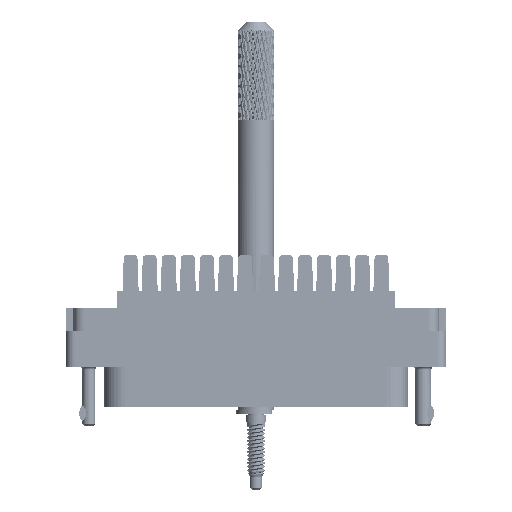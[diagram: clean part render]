
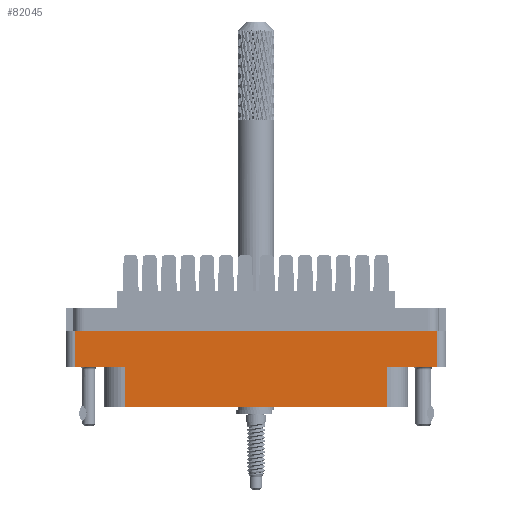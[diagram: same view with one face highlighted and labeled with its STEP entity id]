
A CAD part, front view. The second image highlights one B-rep face of the part: STEP entity #82045.
In plain terms, the highlighted planar face has unit normal (0, -1, 0).
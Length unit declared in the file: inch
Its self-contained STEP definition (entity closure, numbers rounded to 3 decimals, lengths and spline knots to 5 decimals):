
#1005 = VECTOR ( 'NONE', #51727, 39.37008 ) ;
#1274 = LINE ( 'NONE', #11987, #2320 ) ;
#1935 = EDGE_CURVE ( 'NONE', #18866, #2703, #26719, .T. ) ;
#2320 = VECTOR ( 'NONE', #117773, 39.37008 ) ;
#2613 = LINE ( 'NONE', #117264, #1005 ) ;
#2703 = VERTEX_POINT ( 'NONE', #40916 ) ;
#7114 = LINE ( 'NONE', #45533, #73201 ) ;
#8499 = EDGE_CURVE ( 'NONE', #58552, #28259, #59011, .T. ) ;
#11987 = CARTESIAN_POINT ( 'NONE',  ( 1.2335, -0.438, -0.789 ) ) ;
#18866 = VERTEX_POINT ( 'NONE', #91129 ) ;
#19092 = ORIENTED_EDGE ( 'NONE', *, *, #102965, .T. ) ;
#21638 = CARTESIAN_POINT ( 'NONE',  ( -0.895, -0.438, -0.789 ) ) ;
#26719 = LINE ( 'NONE', #103529, #117432 ) ;
#27551 = CARTESIAN_POINT ( 'NONE',  ( 0.895, -0.438, -0.789 ) ) ;
#27897 = EDGE_CURVE ( 'NONE', #28259, #73097, #7114, .T. ) ;
#28191 = CARTESIAN_POINT ( 'NONE',  ( -1.2955, -0.438, -0.789 ) ) ;
#28259 = VERTEX_POINT ( 'NONE', #27551 ) ;
#28790 = CARTESIAN_POINT ( 'NONE',  ( 0.895, -0.438, -0.52 ) ) ;
#29815 = CARTESIAN_POINT ( 'NONE',  ( 0., -0.438, -0.52 ) ) ;
#31301 = VECTOR ( 'NONE', #110032, 39.37008 ) ;
#34337 = DIRECTION ( 'NONE',  ( 0., 0., -1. ) ) ;
#34468 = CARTESIAN_POINT ( 'NONE',  ( 0., -0.438, -0.52 ) ) ;
#40916 = CARTESIAN_POINT ( 'NONE',  ( -1.2335, -0.438, -0.52 ) ) ;
#41035 = CARTESIAN_POINT ( 'NONE',  ( 1.2335, -0.438, -0.274 ) ) ;
#41546 = PLANE ( 'NONE',  #57138 ) ;
#42631 = VERTEX_POINT ( 'NONE', #104382 ) ;
#43410 = DIRECTION ( 'NONE',  ( 0., -1., 0. ) ) ;
#43497 = CARTESIAN_POINT ( 'NONE',  ( -0.895, -0.438, -0.52 ) ) ;
#44516 = EDGE_CURVE ( 'NONE', #42631, #73097, #60889, .T. ) ;
#45533 = CARTESIAN_POINT ( 'NONE',  ( 0.895, -0.438, -0.52 ) ) ;
#48310 = VERTEX_POINT ( 'NONE', #43497 ) ;
#51727 = DIRECTION ( 'NONE',  ( 0., 0., -1. ) ) ;
#52726 = ORIENTED_EDGE ( 'NONE', *, *, #44516, .F. ) ;
#56872 = DIRECTION ( 'NONE',  ( -1., 0., 0. ) ) ;
#57138 = AXIS2_PLACEMENT_3D ( 'NONE', #100698, #43410, #63506 ) ;
#58552 = VERTEX_POINT ( 'NONE', #21638 ) ;
#59011 = LINE ( 'NONE', #28191, #61740 ) ;
#60889 = LINE ( 'NONE', #34468, #83543 ) ;
#61740 = VECTOR ( 'NONE', #105005, 39.37008 ) ;
#62078 = EDGE_CURVE ( 'NONE', #48310, #2703, #65677, .T. ) ;
#62888 = FACE_OUTER_BOUND ( 'NONE', #69247, .T. ) ;
#63506 = DIRECTION ( 'NONE',  ( 0., 0., -1. ) ) ;
#63983 = LINE ( 'NONE', #120758, #31301 ) ;
#65677 = LINE ( 'NONE', #29815, #103940 ) ;
#69247 = EDGE_LOOP ( 'NONE', ( #79613, #100875, #84808, #85115, #98885, #109109, #52726, #19092 ) ) ;
#73097 = VERTEX_POINT ( 'NONE', #28790 ) ;
#73201 = VECTOR ( 'NONE', #83856, 39.37008 ) ;
#79613 = ORIENTED_EDGE ( 'NONE', *, *, #86207, .F. ) ;
#82045 = ADVANCED_FACE ( 'NONE', ( #62888 ), #41546, .T. ) ;
#83543 = VECTOR ( 'NONE', #108162, 39.37008 ) ;
#83856 = DIRECTION ( 'NONE',  ( 0., 0., 1. ) ) ;
#84808 = ORIENTED_EDGE ( 'NONE', *, *, #62078, .F. ) ;
#85115 = ORIENTED_EDGE ( 'NONE', *, *, #108695, .T. ) ;
#86207 = EDGE_CURVE ( 'NONE', #18866, #88969, #63983, .T. ) ;
#88969 = VERTEX_POINT ( 'NONE', #41035 ) ;
#91129 = CARTESIAN_POINT ( 'NONE',  ( -1.2335, -0.438, -0.274 ) ) ;
#98885 = ORIENTED_EDGE ( 'NONE', *, *, #8499, .T. ) ;
#100698 = CARTESIAN_POINT ( 'NONE',  ( -1.2955, -0.438, -0.789 ) ) ;
#100875 = ORIENTED_EDGE ( 'NONE', *, *, #1935, .T. ) ;
#102965 = EDGE_CURVE ( 'NONE', #42631, #88969, #1274, .T. ) ;
#103529 = CARTESIAN_POINT ( 'NONE',  ( -1.2335, -0.438, -0.789 ) ) ;
#103940 = VECTOR ( 'NONE', #56872, 39.37008 ) ;
#104382 = CARTESIAN_POINT ( 'NONE',  ( 1.2335, -0.438, -0.52 ) ) ;
#105005 = DIRECTION ( 'NONE',  ( 1., 0., 0. ) ) ;
#108162 = DIRECTION ( 'NONE',  ( -1., 0., 0. ) ) ;
#108695 = EDGE_CURVE ( 'NONE', #48310, #58552, #2613, .T. ) ;
#109109 = ORIENTED_EDGE ( 'NONE', *, *, #27897, .T. ) ;
#110032 = DIRECTION ( 'NONE',  ( 1., 0., 0. ) ) ;
#117264 = CARTESIAN_POINT ( 'NONE',  ( -0.895, -0.438, -0.789 ) ) ;
#117432 = VECTOR ( 'NONE', #34337, 39.37008 ) ;
#117773 = DIRECTION ( 'NONE',  ( 0., 0., 1. ) ) ;
#120758 = CARTESIAN_POINT ( 'NONE',  ( 0., -0.438, -0.274 ) ) ;
